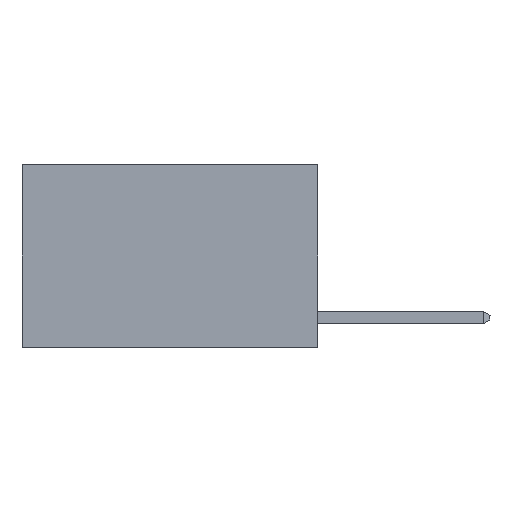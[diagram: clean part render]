
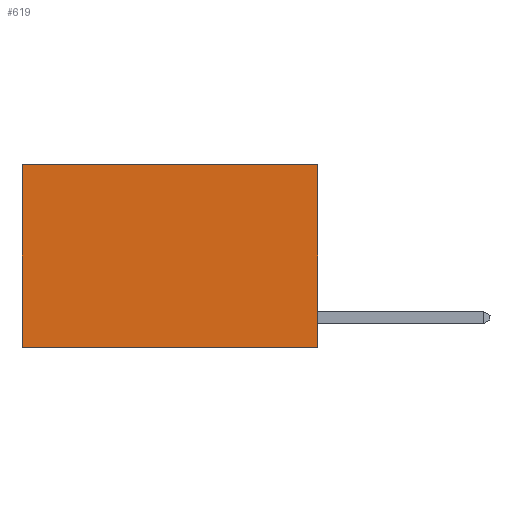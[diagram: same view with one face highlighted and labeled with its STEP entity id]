
A CAD part, left-side view. The second image highlights one B-rep face of the part: STEP entity #619.
In plain terms, the highlighted planar face has unit normal (-1, 0, 0).
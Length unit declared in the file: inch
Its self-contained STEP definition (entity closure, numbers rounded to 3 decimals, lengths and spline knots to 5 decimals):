
#496 = VERTEX_POINT ( 'NONE', #11323 ) ;
#619 = ADVANCED_FACE ( 'NONE', ( #10960 ), #15116, .F. ) ;
#1328 = ORIENTED_EDGE ( 'NONE', *, *, #10913, .F. ) ;
#1661 = DIRECTION ( 'NONE',  ( 0., 0., -1. ) ) ;
#1934 = EDGE_CURVE ( 'NONE', #15577, #496, #13838, .T. ) ;
#2727 = ORIENTED_EDGE ( 'NONE', *, *, #6037, .T. ) ;
#3332 = LINE ( 'NONE', #8466, #7817 ) ;
#3673 = VECTOR ( 'NONE', #15859, 39.37008 ) ;
#5654 = DIRECTION ( 'NONE',  ( 1., 0., 0. ) ) ;
#5674 = VERTEX_POINT ( 'NONE', #15191 ) ;
#6037 = EDGE_CURVE ( 'NONE', #15577, #10795, #15386, .T. ) ;
#6546 = CARTESIAN_POINT ( 'NONE',  ( 0.2625, 0.6, 0. ) ) ;
#7817 = VECTOR ( 'NONE', #8349, 39.37008 ) ;
#8332 = CARTESIAN_POINT ( 'NONE',  ( 0.2625, 0., 0. ) ) ;
#8349 = DIRECTION ( 'NONE',  ( 0., 1., 0. ) ) ;
#8466 = CARTESIAN_POINT ( 'NONE',  ( 0.2625, 0., -0.37 ) ) ;
#8595 = AXIS2_PLACEMENT_3D ( 'NONE', #8332, #5654, #1661 ) ;
#10232 = DIRECTION ( 'NONE',  ( 0., 1., 0. ) ) ;
#10302 = EDGE_CURVE ( 'NONE', #10795, #5674, #14160, .T. ) ;
#10351 = CARTESIAN_POINT ( 'NONE',  ( 0.2625, 0., 0. ) ) ;
#10523 = CARTESIAN_POINT ( 'NONE',  ( 0.2625, 0.6, 0. ) ) ;
#10551 = DIRECTION ( 'NONE',  ( 0., 0., -1. ) ) ;
#10795 = VERTEX_POINT ( 'NONE', #10523 ) ;
#10913 = EDGE_CURVE ( 'NONE', #496, #5674, #3332, .T. ) ;
#10960 = FACE_OUTER_BOUND ( 'NONE', #15602, .T. ) ;
#11323 = CARTESIAN_POINT ( 'NONE',  ( 0.2625, 0., -0.37 ) ) ;
#11802 = VECTOR ( 'NONE', #10232, 39.37008 ) ;
#13784 = ORIENTED_EDGE ( 'NONE', *, *, #10302, .T. ) ;
#13838 = LINE ( 'NONE', #10351, #3673 ) ;
#14160 = LINE ( 'NONE', #6546, #17153 ) ;
#14924 = CARTESIAN_POINT ( 'NONE',  ( 0.2625, 0., 0. ) ) ;
#15116 = PLANE ( 'NONE',  #8595 ) ;
#15191 = CARTESIAN_POINT ( 'NONE',  ( 0.2625, 0.6, -0.37 ) ) ;
#15386 = LINE ( 'NONE', #15497, #11802 ) ;
#15497 = CARTESIAN_POINT ( 'NONE',  ( 0.2625, 0., 0. ) ) ;
#15577 = VERTEX_POINT ( 'NONE', #14924 ) ;
#15602 = EDGE_LOOP ( 'NONE', ( #13784, #1328, #16712, #2727 ) ) ;
#15859 = DIRECTION ( 'NONE',  ( 0., 0., -1. ) ) ;
#16712 = ORIENTED_EDGE ( 'NONE', *, *, #1934, .F. ) ;
#17153 = VECTOR ( 'NONE', #10551, 39.37008 ) ;
